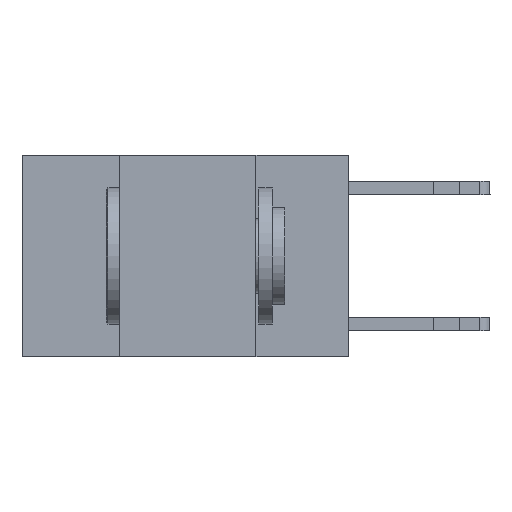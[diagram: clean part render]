
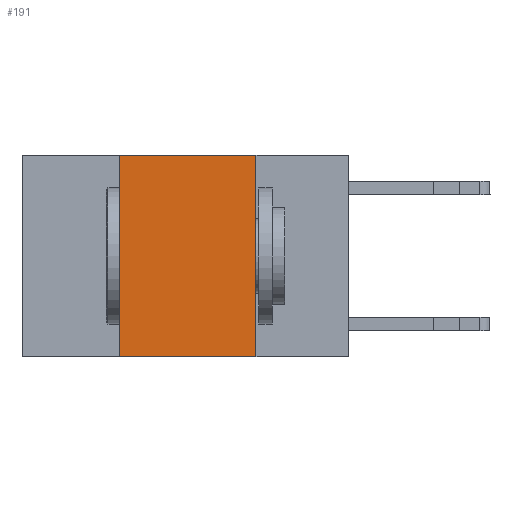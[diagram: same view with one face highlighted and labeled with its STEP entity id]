
A CAD part, left-side view. The second image highlights one B-rep face of the part: STEP entity #191.
In plain terms, the highlighted planar face has unit normal (-1, 0, 0).
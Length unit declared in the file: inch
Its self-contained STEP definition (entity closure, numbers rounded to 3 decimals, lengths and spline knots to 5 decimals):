
#191 = ADVANCED_FACE ( 'NONE', ( #10213 ), #6239, .F. ) ;
#1576 = EDGE_LOOP ( 'NONE', ( #2074, #2545, #2572, #2878 ) ) ;
#2074 = ORIENTED_EDGE ( 'NONE', *, *, #5942, .F. ) ;
#2545 = ORIENTED_EDGE ( 'NONE', *, *, #15781, .F. ) ;
#2572 = ORIENTED_EDGE ( 'NONE', *, *, #7145, .F. ) ;
#2826 = VECTOR ( 'NONE', #18010, 39.37008 ) ;
#2865 = LINE ( 'NONE', #18160, #2826 ) ;
#2878 = ORIENTED_EDGE ( 'NONE', *, *, #22229, .T. ) ;
#3145 = VERTEX_POINT ( 'NONE', #13425 ) ;
#4150 = CARTESIAN_POINT ( 'NONE',  ( 0., 0.17, -0.37 ) ) ;
#4353 = DIRECTION ( 'NONE',  ( 0., 0., 1. ) ) ;
#5098 = DIRECTION ( 'NONE',  ( 1., 0., 0. ) ) ;
#5832 = CARTESIAN_POINT ( 'NONE',  ( 0., 0.42, 0. ) ) ;
#5942 = EDGE_CURVE ( 'NONE', #3145, #11469, #16121, .T. ) ;
#5982 = CARTESIAN_POINT ( 'NONE',  ( 0., 0.42, 0. ) ) ;
#6239 = PLANE ( 'NONE',  #6839 ) ;
#6839 = AXIS2_PLACEMENT_3D ( 'NONE', #12151, #5098, #13918 ) ;
#7145 = EDGE_CURVE ( 'NONE', #9313, #12744, #8658, .T. ) ;
#8543 = VECTOR ( 'NONE', #4353, 39.37008 ) ;
#8658 = LINE ( 'NONE', #5982, #8543 ) ;
#9061 = DIRECTION ( 'NONE',  ( 0., -1., 0. ) ) ;
#9313 = VERTEX_POINT ( 'NONE', #19658 ) ;
#10213 = FACE_OUTER_BOUND ( 'NONE', #1576, .T. ) ;
#11469 = VERTEX_POINT ( 'NONE', #4150 ) ;
#12151 = CARTESIAN_POINT ( 'NONE',  ( 0., 0.6, 0. ) ) ;
#12744 = VERTEX_POINT ( 'NONE', #5832 ) ;
#13425 = CARTESIAN_POINT ( 'NONE',  ( 0., 0.17, 0. ) ) ;
#13918 = DIRECTION ( 'NONE',  ( 0., 0., -1. ) ) ;
#13936 = VECTOR ( 'NONE', #9061, 39.37008 ) ;
#14914 = LINE ( 'NONE', #19348, #13936 ) ;
#15107 = DIRECTION ( 'NONE',  ( 0., 0., -1. ) ) ;
#15428 = CARTESIAN_POINT ( 'NONE',  ( 0., 0.17, 0. ) ) ;
#15781 = EDGE_CURVE ( 'NONE', #12744, #3145, #2865, .T. ) ;
#15976 = VECTOR ( 'NONE', #15107, 39.37008 ) ;
#16121 = LINE ( 'NONE', #15428, #15976 ) ;
#18010 = DIRECTION ( 'NONE',  ( 0., -1., 0. ) ) ;
#18160 = CARTESIAN_POINT ( 'NONE',  ( 0., 0.6, 0. ) ) ;
#19348 = CARTESIAN_POINT ( 'NONE',  ( 0., 0.6, -0.37 ) ) ;
#19658 = CARTESIAN_POINT ( 'NONE',  ( 0., 0.42, -0.37 ) ) ;
#22229 = EDGE_CURVE ( 'NONE', #9313, #11469, #14914, .T. ) ;
